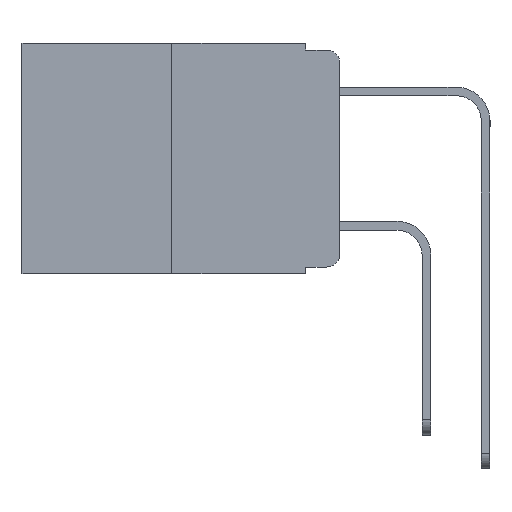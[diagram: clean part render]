
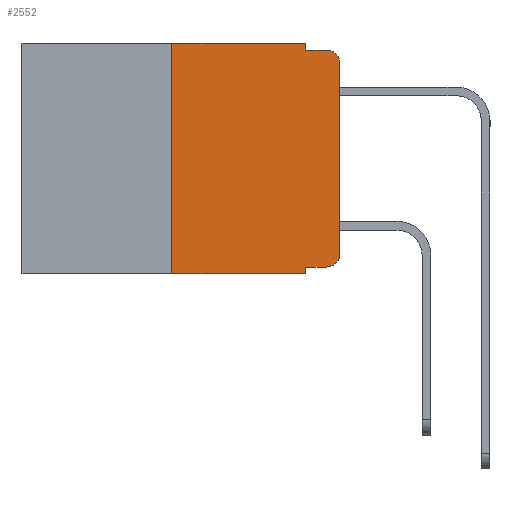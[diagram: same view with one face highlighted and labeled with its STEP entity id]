
A CAD part, left-side view. The second image highlights one B-rep face of the part: STEP entity #2552.
In plain terms, the highlighted planar face has unit normal (-1, 0, 0).
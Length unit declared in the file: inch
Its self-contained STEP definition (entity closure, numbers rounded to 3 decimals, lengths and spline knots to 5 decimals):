
#5 = EDGE_LOOP ( 'NONE', ( #12407, #244, #354, #703, #731, #883, #1002, #1206, #1529, #1537 ) ) ;
#22 = EDGE_CURVE ( 'NONE', #10340, #5756, #865, .T. ) ;
#244 = ORIENTED_EDGE ( 'NONE', *, *, #12151, .T. ) ;
#354 = ORIENTED_EDGE ( 'NONE', *, *, #10112, .F. ) ;
#703 = ORIENTED_EDGE ( 'NONE', *, *, #7360, .F. ) ;
#731 = ORIENTED_EDGE ( 'NONE', *, *, #9970, .F. ) ;
#865 = LINE ( 'NONE', #8728, #11804 ) ;
#883 = ORIENTED_EDGE ( 'NONE', *, *, #6003, .F. ) ;
#1002 = ORIENTED_EDGE ( 'NONE', *, *, #22, .T. ) ;
#1070 = LINE ( 'NONE', #9907, #9629 ) ;
#1206 = ORIENTED_EDGE ( 'NONE', *, *, #4648, .F. ) ;
#1504 = CIRCLE ( 'NONE', #7958, 0.02 ) ;
#1529 = ORIENTED_EDGE ( 'NONE', *, *, #3243, .T. ) ;
#1537 = ORIENTED_EDGE ( 'NONE', *, *, #2563, .T. ) ;
#1623 = CARTESIAN_POINT ( 'NONE',  ( 0., 0.051, -0.01 ) ) ;
#1888 = VERTEX_POINT ( 'NONE', #3528 ) ;
#1980 = VECTOR ( 'NONE', #4182, 39.37008 ) ;
#2420 = DIRECTION ( 'NONE',  ( 0., -1., 0. ) ) ;
#2552 = ADVANCED_FACE ( 'NONE', ( #7745 ), #12926, .F. ) ;
#2563 = EDGE_CURVE ( 'NONE', #7200, #11202, #10477, .T. ) ;
#3098 = VERTEX_POINT ( 'NONE', #1623 ) ;
#3243 = EDGE_CURVE ( 'NONE', #6442, #7200, #10287, .T. ) ;
#3252 = VECTOR ( 'NONE', #12853, 39.37008 ) ;
#3331 = DIRECTION ( 'NONE',  ( -1., 0., 0. ) ) ;
#3528 = CARTESIAN_POINT ( 'NONE',  ( 0., 0.02, -0.01 ) ) ;
#3807 = CARTESIAN_POINT ( 'NONE',  ( 0., 0.051, -0.343 ) ) ;
#4098 = DIRECTION ( 'NONE',  ( 0., -1., 0. ) ) ;
#4173 = CARTESIAN_POINT ( 'NONE',  ( 0., 0.25, 0. ) ) ;
#4182 = DIRECTION ( 'NONE',  ( 0., 0., 1. ) ) ;
#4648 = EDGE_CURVE ( 'NONE', #6442, #5756, #10067, .T. ) ;
#4722 = CARTESIAN_POINT ( 'NONE',  ( 0., 0., -0.03 ) ) ;
#4825 = DIRECTION ( 'NONE',  ( 0., -1., 0. ) ) ;
#4921 = CARTESIAN_POINT ( 'NONE',  ( 0., 0.051, -0.333 ) ) ;
#4993 = LINE ( 'NONE', #6055, #12472 ) ;
#5146 = VERTEX_POINT ( 'NONE', #4722 ) ;
#5369 = DIRECTION ( 'NONE',  ( -1., 0., 0. ) ) ;
#5756 = VERTEX_POINT ( 'NONE', #3807 ) ;
#6003 = EDGE_CURVE ( 'NONE', #10340, #10856, #13027, .T. ) ;
#6055 = CARTESIAN_POINT ( 'NONE',  ( 0., 0.051, -0.01 ) ) ;
#6442 = VERTEX_POINT ( 'NONE', #4921 ) ;
#7056 = AXIS2_PLACEMENT_3D ( 'NONE', #11317, #3331, #12764 ) ;
#7200 = VERTEX_POINT ( 'NONE', #10615 ) ;
#7266 = CARTESIAN_POINT ( 'NONE',  ( 0., 0.25, 0. ) ) ;
#7330 = VECTOR ( 'NONE', #13118, 39.37008 ) ;
#7360 = EDGE_CURVE ( 'NONE', #11728, #3098, #9041, .T. ) ;
#7558 = VECTOR ( 'NONE', #4098, 39.37008 ) ;
#7621 = VECTOR ( 'NONE', #11388, 39.37008 ) ;
#7745 = FACE_OUTER_BOUND ( 'NONE', #5, .T. ) ;
#7753 = AXIS2_PLACEMENT_3D ( 'NONE', #11008, #11773, #11780 ) ;
#7796 = CARTESIAN_POINT ( 'NONE',  ( 0., 0.051, 0. ) ) ;
#7923 = CARTESIAN_POINT ( 'NONE',  ( 0., 0., -0.313 ) ) ;
#7958 = AXIS2_PLACEMENT_3D ( 'NONE', #11467, #5369, #12469 ) ;
#8728 = CARTESIAN_POINT ( 'NONE',  ( 0., 0.473, -0.343 ) ) ;
#9041 = LINE ( 'NONE', #7796, #3252 ) ;
#9629 = VECTOR ( 'NONE', #4825, 39.37008 ) ;
#9907 = CARTESIAN_POINT ( 'NONE',  ( 0., 0.473, 0. ) ) ;
#9970 = EDGE_CURVE ( 'NONE', #10856, #11728, #1070, .T. ) ;
#10067 = LINE ( 'NONE', #12122, #7330 ) ;
#10112 = EDGE_CURVE ( 'NONE', #3098, #1888, #4993, .T. ) ;
#10287 = LINE ( 'NONE', #12392, #7558 ) ;
#10340 = VERTEX_POINT ( 'NONE', #12465 ) ;
#10477 = CIRCLE ( 'NONE', #7056, 0.02 ) ;
#10615 = CARTESIAN_POINT ( 'NONE',  ( 0., 0.02, -0.333 ) ) ;
#10856 = VERTEX_POINT ( 'NONE', #4173 ) ;
#11008 = CARTESIAN_POINT ( 'NONE',  ( 0., 0.473, 0. ) ) ;
#11202 = VERTEX_POINT ( 'NONE', #7923 ) ;
#11314 = CARTESIAN_POINT ( 'NONE',  ( 0., 0., 0. ) ) ;
#11317 = CARTESIAN_POINT ( 'NONE',  ( 0., 0.02, -0.313 ) ) ;
#11388 = DIRECTION ( 'NONE',  ( 0., 0., 1. ) ) ;
#11467 = CARTESIAN_POINT ( 'NONE',  ( 0., 0.02, -0.03 ) ) ;
#11728 = VERTEX_POINT ( 'NONE', #12776 ) ;
#11773 = DIRECTION ( 'NONE',  ( 1., 0., 0. ) ) ;
#11780 = DIRECTION ( 'NONE',  ( 0., 0., -1. ) ) ;
#11804 = VECTOR ( 'NONE', #2420, 39.37008 ) ;
#11933 = LINE ( 'NONE', #11314, #1980 ) ;
#12122 = CARTESIAN_POINT ( 'NONE',  ( 0., 0.051, 0. ) ) ;
#12151 = EDGE_CURVE ( 'NONE', #5146, #1888, #1504, .T. ) ;
#12392 = CARTESIAN_POINT ( 'NONE',  ( 0., 0.051, -0.333 ) ) ;
#12407 = ORIENTED_EDGE ( 'NONE', *, *, #12820, .T. ) ;
#12465 = CARTESIAN_POINT ( 'NONE',  ( 0., 0.25, -0.343 ) ) ;
#12469 = DIRECTION ( 'NONE',  ( 0., 0., -1. ) ) ;
#12472 = VECTOR ( 'NONE', #13162, 39.37008 ) ;
#12764 = DIRECTION ( 'NONE',  ( 0., 0., -1. ) ) ;
#12776 = CARTESIAN_POINT ( 'NONE',  ( 0., 0.051, 0. ) ) ;
#12820 = EDGE_CURVE ( 'NONE', #11202, #5146, #11933, .T. ) ;
#12853 = DIRECTION ( 'NONE',  ( 0., 0., -1. ) ) ;
#12926 = PLANE ( 'NONE',  #7753 ) ;
#13027 = LINE ( 'NONE', #7266, #7621 ) ;
#13118 = DIRECTION ( 'NONE',  ( 0., 0., -1. ) ) ;
#13162 = DIRECTION ( 'NONE',  ( 0., -1., 0. ) ) ;
